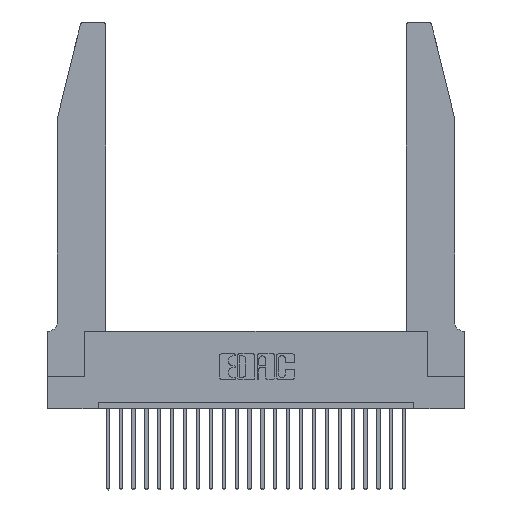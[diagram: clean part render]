
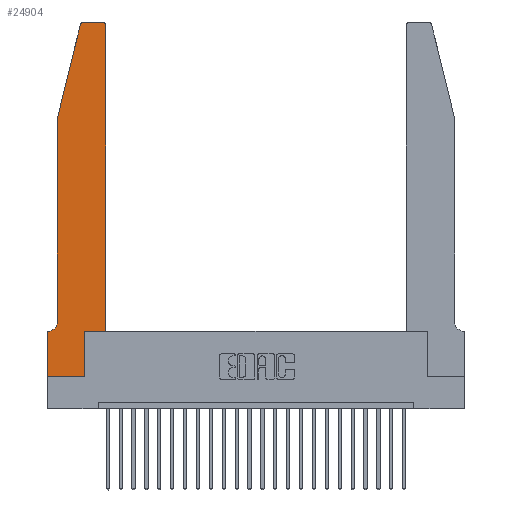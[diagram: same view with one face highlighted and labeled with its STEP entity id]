
A CAD part, top view. The second image highlights one B-rep face of the part: STEP entity #24904.
In plain terms, the highlighted planar face has unit normal (0, 0, 1).
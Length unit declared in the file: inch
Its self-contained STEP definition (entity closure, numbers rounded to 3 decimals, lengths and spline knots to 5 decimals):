
#79 = EDGE_CURVE ( 'NONE', #14821, #13138, #974, .T. ) ;
#724 = DIRECTION ( 'NONE',  ( 0., 0., 1. ) ) ;
#974 = LINE ( 'NONE', #1457, #14695 ) ;
#1457 = CARTESIAN_POINT ( 'NONE',  ( 0.4505, 0.35, 0.37 ) ) ;
#1521 = VERTEX_POINT ( 'NONE', #2934 ) ;
#1793 = EDGE_CURVE ( 'NONE', #2769, #10779, #15825, .T. ) ;
#1971 = ORIENTED_EDGE ( 'NONE', *, *, #21920, .T. ) ;
#2011 = LINE ( 'NONE', #13203, #21202 ) ;
#2061 = VERTEX_POINT ( 'NONE', #9412 ) ;
#2106 = ORIENTED_EDGE ( 'NONE', *, *, #14476, .T. ) ;
#2205 = CARTESIAN_POINT ( 'NONE',  ( 0.284, 2.75, 0.37 ) ) ;
#2514 = CARTESIAN_POINT ( 'NONE',  ( 0., 0.35, 0.37 ) ) ;
#2769 = VERTEX_POINT ( 'NONE', #2205 ) ;
#2934 = CARTESIAN_POINT ( 'NONE',  ( 0., 0., 0.37 ) ) ;
#3092 = AXIS2_PLACEMENT_3D ( 'NONE', #17623, #9695, #23536 ) ;
#3452 = ORIENTED_EDGE ( 'NONE', *, *, #15455, .T. ) ;
#3483 = CARTESIAN_POINT ( 'NONE',  ( 0.4205, 2.72, 0.37 ) ) ;
#3513 = CIRCLE ( 'NONE', #18062, 0.03 ) ;
#4269 = LINE ( 'NONE', #11046, #21361 ) ;
#4348 = CARTESIAN_POINT ( 'NONE',  ( 0.4505, 0.35, 0.37 ) ) ;
#4525 = CARTESIAN_POINT ( 'NONE',  ( 0.2605, 2.75, 0.37 ) ) ;
#4827 = DIRECTION ( 'NONE',  ( -1., 0., 0. ) ) ;
#5383 = CARTESIAN_POINT ( 'NONE',  ( 0.4505, 2.72, 0.37 ) ) ;
#5742 = EDGE_CURVE ( 'NONE', #13138, #18647, #15482, .T. ) ;
#6062 = EDGE_CURVE ( 'NONE', #17383, #1521, #14043, .T. ) ;
#6786 = DIRECTION ( 'NONE',  ( 0., -1., 0. ) ) ;
#6843 = VECTOR ( 'NONE', #6786, 39.37008 ) ;
#7064 = DIRECTION ( 'NONE',  ( -0.239, -0.971, 0. ) ) ;
#7098 = ORIENTED_EDGE ( 'NONE', *, *, #1793, .T. ) ;
#8683 = CARTESIAN_POINT ( 'NONE',  ( 0., 0., 0.37 ) ) ;
#8892 = CARTESIAN_POINT ( 'NONE',  ( 0.0755, 2., 0.37 ) ) ;
#9375 = DIRECTION ( 'NONE',  ( 1., 0., 0. ) ) ;
#9412 = CARTESIAN_POINT ( 'NONE',  ( 0.4205, 2.75, 0.37 ) ) ;
#9695 = DIRECTION ( 'NONE',  ( 0., 0., 1. ) ) ;
#9993 = VECTOR ( 'NONE', #14584, 39.37008 ) ;
#10253 = LINE ( 'NONE', #19100, #14539 ) ;
#10361 = ORIENTED_EDGE ( 'NONE', *, *, #5742, .T. ) ;
#10659 = CARTESIAN_POINT ( 'NONE',  ( 0.0755, 0.35, 0.37 ) ) ;
#10779 = VERTEX_POINT ( 'NONE', #14106 ) ;
#11012 = CARTESIAN_POINT ( 'NONE',  ( 0., 0.35, 0.37 ) ) ;
#11046 = CARTESIAN_POINT ( 'NONE',  ( 0.0755, 2., 0.37 ) ) ;
#11328 = VECTOR ( 'NONE', #4827, 39.37008 ) ;
#11530 = ORIENTED_EDGE ( 'NONE', *, *, #6062, .T. ) ;
#11797 = VECTOR ( 'NONE', #17982, 39.37008 ) ;
#12544 = CARTESIAN_POINT ( 'NONE',  ( 0.0755, 2., 0.37 ) ) ;
#12558 = ORIENTED_EDGE ( 'NONE', *, *, #19767, .T. ) ;
#12779 = VERTEX_POINT ( 'NONE', #16333 ) ;
#12786 = ORIENTED_EDGE ( 'NONE', *, *, #79, .T. ) ;
#13138 = VERTEX_POINT ( 'NONE', #22268 ) ;
#13203 = CARTESIAN_POINT ( 'NONE',  ( 0.2865, 0.35, 0.37 ) ) ;
#13439 = ORIENTED_EDGE ( 'NONE', *, *, #15007, .T. ) ;
#14043 = LINE ( 'NONE', #8683, #19242 ) ;
#14106 = CARTESIAN_POINT ( 'NONE',  ( 0.25487, 2.72718, 0.37 ) ) ;
#14476 = EDGE_CURVE ( 'NONE', #1521, #12779, #10253, .T. ) ;
#14539 = VECTOR ( 'NONE', #9375, 39.37008 ) ;
#14584 = DIRECTION ( 'NONE',  ( -1., 0., 0. ) ) ;
#14695 = VECTOR ( 'NONE', #14823, 39.37008 ) ;
#14821 = VERTEX_POINT ( 'NONE', #14915 ) ;
#14823 = DIRECTION ( 'NONE',  ( 1., 0., 0. ) ) ;
#14915 = CARTESIAN_POINT ( 'NONE',  ( 0.2865, 0.35, 0.37 ) ) ;
#15007 = EDGE_CURVE ( 'NONE', #23967, #24354, #19683, .T. ) ;
#15225 = ORIENTED_EDGE ( 'NONE', *, *, #23079, .T. ) ;
#15455 = EDGE_CURVE ( 'NONE', #12779, #14821, #2011, .T. ) ;
#15482 = LINE ( 'NONE', #4348, #11797 ) ;
#15825 = CIRCLE ( 'NONE', #3092, 0.03 ) ;
#15949 = ORIENTED_EDGE ( 'NONE', *, *, #22095, .T. ) ;
#16333 = CARTESIAN_POINT ( 'NONE',  ( 0.2865, 0., 0.37 ) ) ;
#17000 = DIRECTION ( 'NONE',  ( 0., 1., 0. ) ) ;
#17383 = VERTEX_POINT ( 'NONE', #11012 ) ;
#17623 = CARTESIAN_POINT ( 'NONE',  ( 0.284, 2.72, 0.37 ) ) ;
#17953 = AXIS2_PLACEMENT_3D ( 'NONE', #24019, #18522, #20223 ) ;
#17982 = DIRECTION ( 'NONE',  ( 0., 1., 0. ) ) ;
#17997 = FACE_OUTER_BOUND ( 'NONE', #21523, .T. ) ;
#18062 = AXIS2_PLACEMENT_3D ( 'NONE', #3483, #19075, #24567 ) ;
#18522 = DIRECTION ( 'NONE',  ( 0., 0., -1. ) ) ;
#18581 = EDGE_CURVE ( 'NONE', #10779, #20825, #4269, .T. ) ;
#18647 = VERTEX_POINT ( 'NONE', #5383 ) ;
#18666 = LINE ( 'NONE', #10659, #11328 ) ;
#19075 = DIRECTION ( 'NONE',  ( 0., 0., 1. ) ) ;
#19100 = CARTESIAN_POINT ( 'NONE',  ( 0., 0., 0.37 ) ) ;
#19242 = VECTOR ( 'NONE', #24292, 39.37008 ) ;
#19683 = CIRCLE ( 'NONE', #17953, 0.07 ) ;
#19767 = EDGE_CURVE ( 'NONE', #2061, #2769, #20047, .T. ) ;
#20047 = LINE ( 'NONE', #4525, #9993 ) ;
#20223 = DIRECTION ( 'NONE',  ( -1., 0., 0. ) ) ;
#20228 = PLANE ( 'NONE',  #23141 ) ;
#20704 = CARTESIAN_POINT ( 'NONE',  ( 0.0055, 0.35, 0.37 ) ) ;
#20825 = VERTEX_POINT ( 'NONE', #8892 ) ;
#21202 = VECTOR ( 'NONE', #17000, 39.37008 ) ;
#21361 = VECTOR ( 'NONE', #7064, 39.37008 ) ;
#21523 = EDGE_LOOP ( 'NONE', ( #12558, #7098, #22765, #1971, #13439, #15225, #11530, #2106, #3452, #12786, #10361, #15949 ) ) ;
#21920 = EDGE_CURVE ( 'NONE', #20825, #23967, #23874, .T. ) ;
#22095 = EDGE_CURVE ( 'NONE', #18647, #2061, #3513, .T. ) ;
#22268 = CARTESIAN_POINT ( 'NONE',  ( 0.4505, 0.35, 0.37 ) ) ;
#22765 = ORIENTED_EDGE ( 'NONE', *, *, #18581, .T. ) ;
#22906 = CARTESIAN_POINT ( 'NONE',  ( 0.0755, 0.42, 0.37 ) ) ;
#23079 = EDGE_CURVE ( 'NONE', #24354, #17383, #18666, .T. ) ;
#23141 = AXIS2_PLACEMENT_3D ( 'NONE', #2514, #724, #23952 ) ;
#23536 = DIRECTION ( 'NONE',  ( 1., 0., 0. ) ) ;
#23874 = LINE ( 'NONE', #12544, #6843 ) ;
#23952 = DIRECTION ( 'NONE',  ( 1., 0., 0. ) ) ;
#23967 = VERTEX_POINT ( 'NONE', #22906 ) ;
#24019 = CARTESIAN_POINT ( 'NONE',  ( 0.0055, 0.42, 0.37 ) ) ;
#24292 = DIRECTION ( 'NONE',  ( 0., -1., 0. ) ) ;
#24354 = VERTEX_POINT ( 'NONE', #20704 ) ;
#24567 = DIRECTION ( 'NONE',  ( 1., 0., 0. ) ) ;
#24904 = ADVANCED_FACE ( 'NONE', ( #17997 ), #20228, .T. ) ;
